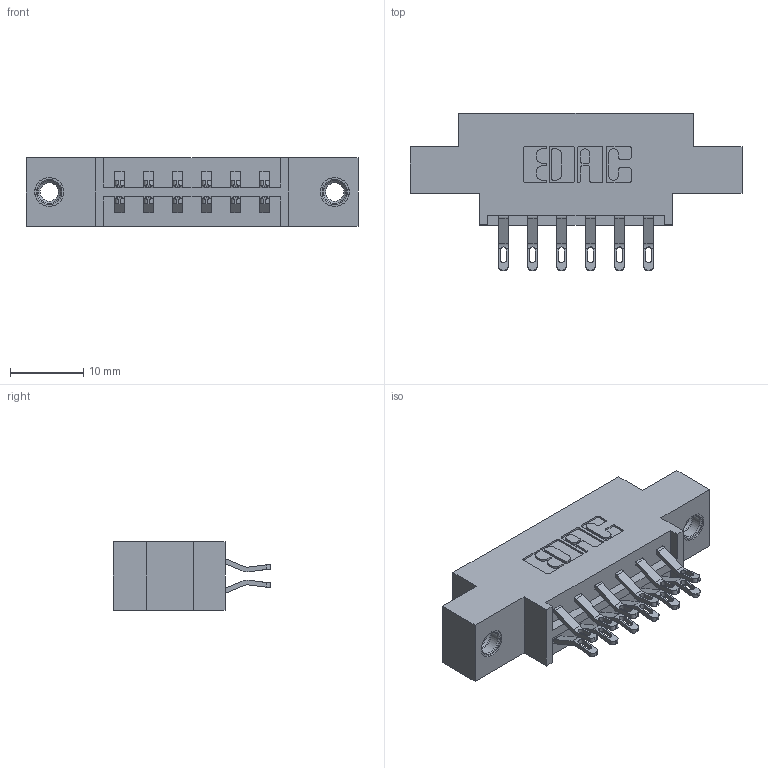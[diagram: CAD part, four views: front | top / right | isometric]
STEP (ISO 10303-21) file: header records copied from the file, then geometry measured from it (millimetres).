
FILE_DESCRIPTION (( 'STEP AP203' ), '1' );
FILE_NAME ('833-012-555-807.STEP', '2020-05-30T22:37:27', ( '' ), ( '' ), 'SwSTEP 2.0', 'SolidWorks 2020', '' );
FILE_SCHEMA (( 'CONFIG_CONTROL_DESIGN' ));
Length unit declared in the file: inch
Products named in the file (4): 833-012-555-807; 345-292-001_555 Tail; 833 Part_Offset - .156 Dia - TI; 345-250-001_345-250-005-103
Assembly tree (15 placements, depth 2):
  833-012-555-807
    833 Part_Offset - .156 Dia - TI
    345-292-001_555 Tail  x12
    345-250-001_345-250-005-103  x2
Bounding box: 45.31 x 21.47 x 9.4 mm (x, y, z)
Volume: 4083.1 mm3; surface area: 4825.5 mm2
Topology: 15 solids, 15 shells, 874 faces, 2655 edges, 1762 vertices
Faces by surface type: plane 514, cylinder 344, cone 12, torus 4
Entity records: 10160 total; most frequent: CARTESIAN_POINT 1747, ORIENTED_EDGE 1646, DIRECTION 1557, EDGE_CURVE 823, LINE 655, VECTOR 655, VERTEX_POINT 544, AXIS2_PLACEMENT_3D 451
